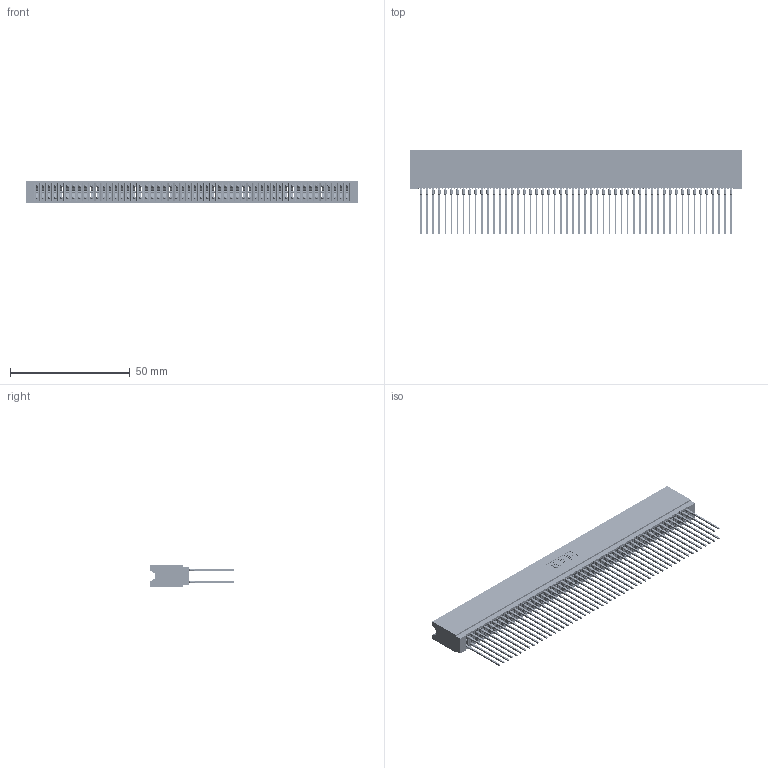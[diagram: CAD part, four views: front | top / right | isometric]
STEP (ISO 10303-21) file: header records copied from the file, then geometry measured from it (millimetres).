
FILE_DESCRIPTION (( 'STEP AP203' ), '1' );
FILE_NAME ('745-104-541-206.STEP', '2026-02-26T23:46:51', ( '' ), ( '' ), 'SwSTEP 2.0', 'SolidWorks 2023', '' );
FILE_SCHEMA (( 'CONFIG_CONTROL_DESIGN' ));
Length unit declared in the file: millimetre
Products named in the file (3): 745-104-541-206; 745-292-001_541; 745 Part_Insulator Option - 06
Assembly tree (105 placements, depth 2):
  745-104-541-206
    745 Part_Insulator Option - 06
    745-292-001_541  x104
Bounding box: 138.68 x 35.45 x 8.89 mm (x, y, z)
Volume: 12916.1 mm3; surface area: 28580.5 mm2
Topology: 105 solids, 105 shells, 9404 faces, 25272 edges, 15876 vertices
Faces by surface type: plane 4840, bspline 2080, cylinder 1860, torus 624
Entity records: 86198 total; most frequent: CARTESIAN_POINT 15450, ORIENTED_EDGE 14906, DIRECTION 13013, EDGE_CURVE 7453, LINE 6959, VECTOR 6959, VERTEX_POINT 4752, AXIS2_PLACEMENT_3D 3027
